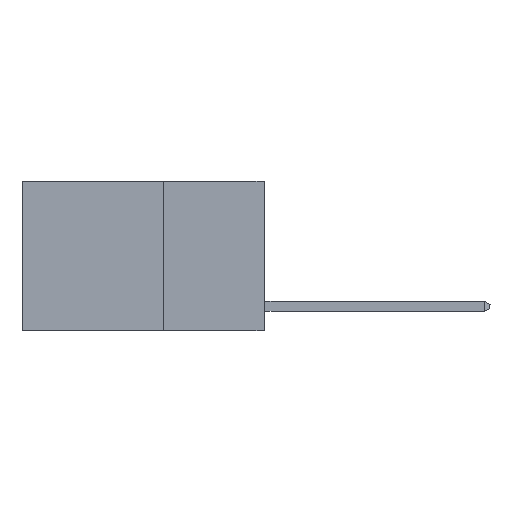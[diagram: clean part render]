
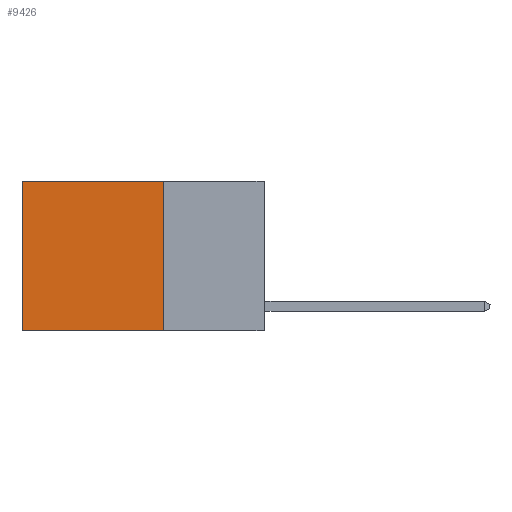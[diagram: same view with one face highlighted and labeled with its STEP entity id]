
A CAD part, left-side view. The second image highlights one B-rep face of the part: STEP entity #9426.
In plain terms, the highlighted planar face has unit normal (-1, 0, 0).
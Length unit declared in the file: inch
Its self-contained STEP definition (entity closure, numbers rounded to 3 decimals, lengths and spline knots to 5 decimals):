
#105 = ORIENTED_EDGE ( 'NONE', *, *, #3169, .F. ) ;
#175 = DIRECTION ( 'NONE',  ( 0., 0., -1. ) ) ;
#243 = VECTOR ( 'NONE', #942, 39.37008 ) ;
#300 = VERTEX_POINT ( 'NONE', #7164 ) ;
#942 = DIRECTION ( 'NONE',  ( 0., 1., 0. ) ) ;
#982 = CARTESIAN_POINT ( 'NONE',  ( 0.2625, 0.25, 0. ) ) ;
#985 = PLANE ( 'NONE',  #4892 ) ;
#1913 = LINE ( 'NONE', #2266, #8438 ) ;
#2266 = CARTESIAN_POINT ( 'NONE',  ( 0.2625, 0.6, 0. ) ) ;
#2358 = VECTOR ( 'NONE', #6215, 39.37008 ) ;
#2362 = DIRECTION ( 'NONE',  ( 0., 0., -1. ) ) ;
#2567 = ORIENTED_EDGE ( 'NONE', *, *, #7210, .T. ) ;
#2839 = DIRECTION ( 'NONE',  ( 0., 1., 0. ) ) ;
#3169 = EDGE_CURVE ( 'NONE', #7805, #10762, #5913, .T. ) ;
#3652 = ORIENTED_EDGE ( 'NONE', *, *, #10837, .T. ) ;
#3966 = CARTESIAN_POINT ( 'NONE',  ( 0.2625, 0.6, -0.37 ) ) ;
#4892 = AXIS2_PLACEMENT_3D ( 'NONE', #7776, #10340, #175 ) ;
#5361 = EDGE_LOOP ( 'NONE', ( #3652, #105, #7983, #2567 ) ) ;
#5415 = FACE_OUTER_BOUND ( 'NONE', #5361, .T. ) ;
#5562 = EDGE_CURVE ( 'NONE', #300, #7805, #9175, .T. ) ;
#5913 = LINE ( 'NONE', #6247, #8297 ) ;
#6215 = DIRECTION ( 'NONE',  ( 0., 0., -1. ) ) ;
#6247 = CARTESIAN_POINT ( 'NONE',  ( 0.2625, 0.25, -0.37 ) ) ;
#7164 = CARTESIAN_POINT ( 'NONE',  ( 0.2625, 0.25, 0. ) ) ;
#7210 = EDGE_CURVE ( 'NONE', #300, #8662, #9432, .T. ) ;
#7776 = CARTESIAN_POINT ( 'NONE',  ( 0.2625, 0.25, 0. ) ) ;
#7805 = VERTEX_POINT ( 'NONE', #8214 ) ;
#7983 = ORIENTED_EDGE ( 'NONE', *, *, #5562, .F. ) ;
#8214 = CARTESIAN_POINT ( 'NONE',  ( 0.2625, 0.25, -0.37 ) ) ;
#8297 = VECTOR ( 'NONE', #2839, 39.37008 ) ;
#8438 = VECTOR ( 'NONE', #2362, 39.37008 ) ;
#8662 = VERTEX_POINT ( 'NONE', #9399 ) ;
#8686 = CARTESIAN_POINT ( 'NONE',  ( 0.2625, 0.25, 0. ) ) ;
#9175 = LINE ( 'NONE', #8686, #2358 ) ;
#9399 = CARTESIAN_POINT ( 'NONE',  ( 0.2625, 0.6, 0. ) ) ;
#9426 = ADVANCED_FACE ( 'NONE', ( #5415 ), #985, .F. ) ;
#9432 = LINE ( 'NONE', #982, #243 ) ;
#10340 = DIRECTION ( 'NONE',  ( 1., 0., 0. ) ) ;
#10762 = VERTEX_POINT ( 'NONE', #3966 ) ;
#10837 = EDGE_CURVE ( 'NONE', #8662, #10762, #1913, .T. ) ;
